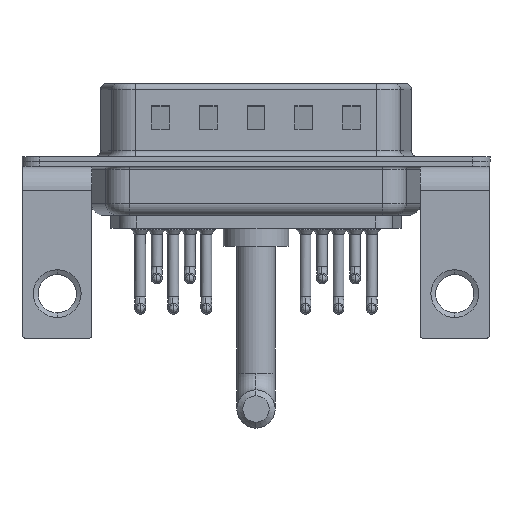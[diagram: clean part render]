
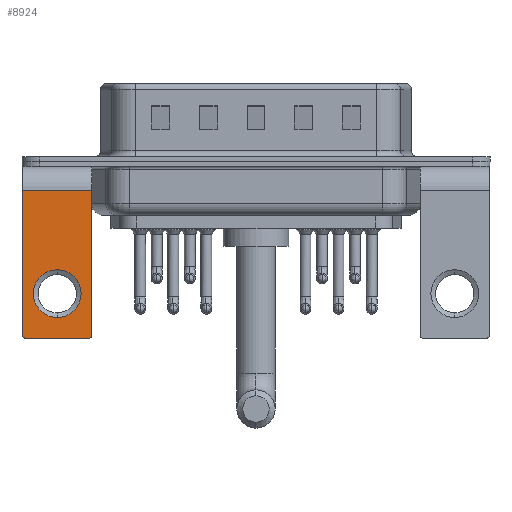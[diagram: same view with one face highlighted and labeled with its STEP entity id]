
A CAD part, front view. The second image highlights one B-rep face of the part: STEP entity #8924.
In plain terms, the highlighted planar face has unit normal (0, -1, 0).
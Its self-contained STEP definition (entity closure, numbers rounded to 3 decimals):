
#834 = VECTOR ( 'NONE', #17001, 1000. ) ;
#875 = CARTESIAN_POINT ( 'NONE',  ( 2.9, -6.25, -14.55 ) ) ;
#1336 = VERTEX_POINT ( 'NONE', #6431 ) ;
#1603 = VERTEX_POINT ( 'NONE', #19267 ) ;
#1915 = CARTESIAN_POINT ( 'NONE',  ( 0., -6.25, -11.07 ) ) ;
#2213 = EDGE_CURVE ( 'NONE', #6100, #5027, #6320, .T. ) ;
#2678 = DIRECTION ( 'NONE',  ( 0., 0., 1. ) ) ;
#2912 = VECTOR ( 'NONE', #20447, 1000. ) ;
#3261 = CARTESIAN_POINT ( 'NONE',  ( 0., -6.25, -11.07 ) ) ;
#3373 = ORIENTED_EDGE ( 'NONE', *, *, #17535, .T. ) ;
#3560 = CARTESIAN_POINT ( 'NONE',  ( 2.9, -6.25, -2.4 ) ) ;
#3862 = VECTOR ( 'NONE', #12090, 1000. ) ;
#4684 = DIRECTION ( 'NONE',  ( 0., -1., 0. ) ) ;
#5027 = VERTEX_POINT ( 'NONE', #875 ) ;
#5355 = FACE_BOUND ( 'NONE', #15337, .T. ) ;
#5359 = DIRECTION ( 'NONE',  ( -1., 0., 0. ) ) ;
#5718 = CARTESIAN_POINT ( 'NONE',  ( 2.9, -6.25, -2.4 ) ) ;
#6100 = VERTEX_POINT ( 'NONE', #23005 ) ;
#6319 = LINE ( 'NONE', #13240, #834 ) ;
#6320 = CIRCLE ( 'NONE', #19423, 0.25 ) ;
#6431 = CARTESIAN_POINT ( 'NONE',  ( 0., -6.25, -9.07 ) ) ;
#6565 = EDGE_CURVE ( 'NONE', #8338, #11380, #22631, .T. ) ;
#6667 = CARTESIAN_POINT ( 'NONE',  ( -2.65, -6.25, -14.55 ) ) ;
#6893 = DIRECTION ( 'NONE',  ( 0., 1., 0. ) ) ;
#7981 = CARTESIAN_POINT ( 'NONE',  ( -2.9, -6.25, -14.55 ) ) ;
#8297 = DIRECTION ( 'NONE',  ( 0., 0., 1. ) ) ;
#8338 = VERTEX_POINT ( 'NONE', #18301 ) ;
#8395 = CARTESIAN_POINT ( 'NONE',  ( 2.9, -6.25, -2.4 ) ) ;
#8529 = DIRECTION ( 'NONE',  ( 0., 0., 1. ) ) ;
#8924 = ADVANCED_FACE ( 'NONE', ( #5355, #14247 ), #17653, .F. ) ;
#9368 = CIRCLE ( 'NONE', #17247, 0.25 ) ;
#10208 = CARTESIAN_POINT ( 'NONE',  ( -2.9, -6.25, -2.4 ) ) ;
#10261 = EDGE_CURVE ( 'NONE', #11380, #1603, #9368, .T. ) ;
#10792 = DIRECTION ( 'NONE',  ( 0., 1., 0. ) ) ;
#11380 = VERTEX_POINT ( 'NONE', #7981 ) ;
#11382 = EDGE_CURVE ( 'NONE', #6100, #1603, #6319, .T. ) ;
#11505 = VERTEX_POINT ( 'NONE', #19220 ) ;
#12090 = DIRECTION ( 'NONE',  ( 0., 0., -1. ) ) ;
#12147 = DIRECTION ( 'NONE',  ( 0., 0., 1. ) ) ;
#12222 = ORIENTED_EDGE ( 'NONE', *, *, #19678, .T. ) ;
#12741 = VERTEX_POINT ( 'NONE', #3560 ) ;
#13240 = CARTESIAN_POINT ( 'NONE',  ( 2.9, -6.25, -14.8 ) ) ;
#13348 = CIRCLE ( 'NONE', #18966, 2. ) ;
#13428 = DIRECTION ( 'NONE',  ( 0., -1., 0. ) ) ;
#14247 = FACE_OUTER_BOUND ( 'NONE', #19505, .T. ) ;
#14422 = DIRECTION ( 'NONE',  ( 0., 0., 1. ) ) ;
#14515 = CIRCLE ( 'NONE', #15276, 2. ) ;
#15072 = LINE ( 'NONE', #5718, #2912 ) ;
#15276 = AXIS2_PLACEMENT_3D ( 'NONE', #3261, #6893, #8297 ) ;
#15314 = CARTESIAN_POINT ( 'NONE',  ( 2.65, -6.25, -14.55 ) ) ;
#15337 = EDGE_LOOP ( 'NONE', ( #12222, #3373 ) ) ;
#16144 = ORIENTED_EDGE ( 'NONE', *, *, #18635, .F. ) ;
#16868 = ORIENTED_EDGE ( 'NONE', *, *, #2213, .T. ) ;
#17001 = DIRECTION ( 'NONE',  ( -1., 0., 0. ) ) ;
#17247 = AXIS2_PLACEMENT_3D ( 'NONE', #6667, #4684, #8529 ) ;
#17535 = EDGE_CURVE ( 'NONE', #1336, #11505, #13348, .T. ) ;
#17610 = VECTOR ( 'NONE', #5359, 1000. ) ;
#17653 = PLANE ( 'NONE',  #22166 ) ;
#18301 = CARTESIAN_POINT ( 'NONE',  ( -2.9, -6.25, -2.4 ) ) ;
#18378 = ORIENTED_EDGE ( 'NONE', *, *, #6565, .T. ) ;
#18635 = EDGE_CURVE ( 'NONE', #12741, #5027, #15072, .T. ) ;
#18883 = ORIENTED_EDGE ( 'NONE', *, *, #21007, .T. ) ;
#18966 = AXIS2_PLACEMENT_3D ( 'NONE', #1915, #10792, #14422 ) ;
#19220 = CARTESIAN_POINT ( 'NONE',  ( 0., -6.25, -13.07 ) ) ;
#19267 = CARTESIAN_POINT ( 'NONE',  ( -2.65, -6.25, -14.8 ) ) ;
#19291 = DIRECTION ( 'NONE',  ( 0., 1., 0. ) ) ;
#19423 = AXIS2_PLACEMENT_3D ( 'NONE', #15314, #13428, #2678 ) ;
#19505 = EDGE_LOOP ( 'NONE', ( #18378, #19751, #19681, #16868, #16144, #18883 ) ) ;
#19678 = EDGE_CURVE ( 'NONE', #11505, #1336, #14515, .T. ) ;
#19681 = ORIENTED_EDGE ( 'NONE', *, *, #11382, .F. ) ;
#19751 = ORIENTED_EDGE ( 'NONE', *, *, #10261, .T. ) ;
#20447 = DIRECTION ( 'NONE',  ( 0., 0., -1. ) ) ;
#21007 = EDGE_CURVE ( 'NONE', #12741, #8338, #21051, .T. ) ;
#21051 = LINE ( 'NONE', #21399, #17610 ) ;
#21399 = CARTESIAN_POINT ( 'NONE',  ( 2.9, -6.25, -2.4 ) ) ;
#22166 = AXIS2_PLACEMENT_3D ( 'NONE', #8395, #19291, #12147 ) ;
#22631 = LINE ( 'NONE', #10208, #3862 ) ;
#23005 = CARTESIAN_POINT ( 'NONE',  ( 2.65, -6.25, -14.8 ) ) ;
